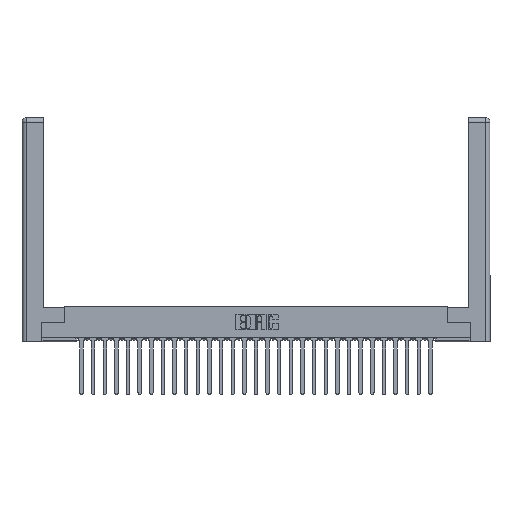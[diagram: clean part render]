
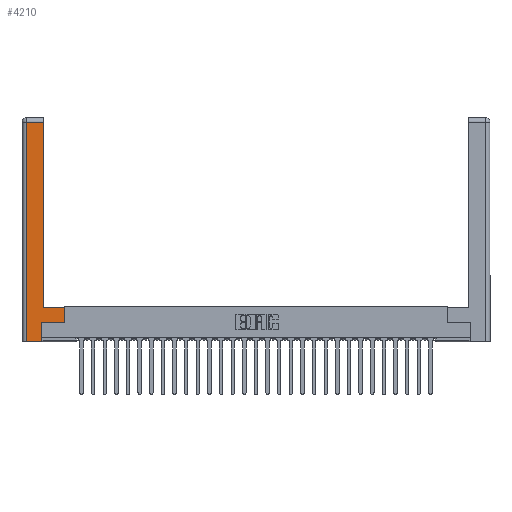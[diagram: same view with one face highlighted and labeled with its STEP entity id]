
A CAD part, top view. The second image highlights one B-rep face of the part: STEP entity #4210.
In plain terms, the highlighted planar face has unit normal (0, 0, 1).
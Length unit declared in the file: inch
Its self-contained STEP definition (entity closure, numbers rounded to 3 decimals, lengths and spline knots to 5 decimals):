
#70 = CARTESIAN_POINT ( 'NONE',  ( 0.265, 0.245, 0. ) ) ;
#2026 = VERTEX_POINT ( 'NONE', #13066 ) ;
#2147 = LINE ( 'NONE', #11250, #27259 ) ;
#2596 = DIRECTION ( 'NONE',  ( -1., 0., 0. ) ) ;
#3195 = ORIENTED_EDGE ( 'NONE', *, *, #26082, .T. ) ;
#3991 = EDGE_CURVE ( 'NONE', #13642, #24415, #12221, .T. ) ;
#4210 = ADVANCED_FACE ( 'NONE', ( #15897 ), #30263, .F. ) ;
#4246 = VECTOR ( 'NONE', #17911, 39.37008 ) ;
#5346 = VECTOR ( 'NONE', #6968, 39.37008 ) ;
#6277 = VERTEX_POINT ( 'NONE', #70 ) ;
#6968 = DIRECTION ( 'NONE',  ( 0., 1., 0. ) ) ;
#7198 = DIRECTION ( 'NONE',  ( 1., 0., 0. ) ) ;
#8032 = EDGE_CURVE ( 'NONE', #24415, #6277, #14075, .T. ) ;
#8377 = VERTEX_POINT ( 'NONE', #27374 ) ;
#8757 = LINE ( 'NONE', #20381, #4246 ) ;
#9289 = CARTESIAN_POINT ( 'NONE',  ( 0.265, 0., 0. ) ) ;
#9421 = VECTOR ( 'NONE', #11457, 39.37008 ) ;
#10796 = ORIENTED_EDGE ( 'NONE', *, *, #13931, .T. ) ;
#11250 = CARTESIAN_POINT ( 'NONE',  ( 0.0615, 0., 0. ) ) ;
#11457 = DIRECTION ( 'NONE',  ( 0., 1., 0. ) ) ;
#12221 = LINE ( 'NONE', #9289, #17261 ) ;
#12653 = VERTEX_POINT ( 'NONE', #21847 ) ;
#12697 = CARTESIAN_POINT ( 'NONE',  ( 0.295, 3., 0. ) ) ;
#12807 = AXIS2_PLACEMENT_3D ( 'NONE', #29969, #27659, #16195 ) ;
#13066 = CARTESIAN_POINT ( 'NONE',  ( 0.295, 2.94, 0. ) ) ;
#13238 = CARTESIAN_POINT ( 'NONE',  ( 0.565, 0.245, 0. ) ) ;
#13642 = VERTEX_POINT ( 'NONE', #19598 ) ;
#13931 = EDGE_CURVE ( 'NONE', #6277, #22882, #23302, .T. ) ;
#14075 = LINE ( 'NONE', #28162, #5346 ) ;
#14352 = VECTOR ( 'NONE', #21273, 39.37008 ) ;
#15060 = EDGE_CURVE ( 'NONE', #12653, #30357, #8757, .T. ) ;
#15392 = ORIENTED_EDGE ( 'NONE', *, *, #19309, .T. ) ;
#15897 = FACE_OUTER_BOUND ( 'NONE', #22704, .T. ) ;
#16195 = DIRECTION ( 'NONE',  ( -1., 0., 0. ) ) ;
#17261 = VECTOR ( 'NONE', #21227, 39.37008 ) ;
#17666 = LINE ( 'NONE', #12697, #14352 ) ;
#17911 = DIRECTION ( 'NONE',  ( -1., 0., 0. ) ) ;
#18518 = ORIENTED_EDGE ( 'NONE', *, *, #15060, .T. ) ;
#18718 = ORIENTED_EDGE ( 'NONE', *, *, #21838, .T. ) ;
#18902 = LINE ( 'NONE', #23404, #9421 ) ;
#19309 = EDGE_CURVE ( 'NONE', #2026, #8377, #23787, .T. ) ;
#19598 = CARTESIAN_POINT ( 'NONE',  ( 0.0615, 0., 0. ) ) ;
#20381 = CARTESIAN_POINT ( 'NONE',  ( 0.295, 0.45, 0. ) ) ;
#20467 = CARTESIAN_POINT ( 'NONE',  ( 0.265, 0., 0. ) ) ;
#21227 = DIRECTION ( 'NONE',  ( 1., 0., 0. ) ) ;
#21273 = DIRECTION ( 'NONE',  ( 0., 1., 0. ) ) ;
#21838 = EDGE_CURVE ( 'NONE', #30357, #2026, #17666, .T. ) ;
#21847 = CARTESIAN_POINT ( 'NONE',  ( 0.565, 0.45, 0. ) ) ;
#22194 = CARTESIAN_POINT ( 'NONE',  ( 0.0615, 2.94, 0. ) ) ;
#22704 = EDGE_LOOP ( 'NONE', ( #18718, #15392, #29010, #28416, #23493, #10796, #3195, #18518 ) ) ;
#22882 = VERTEX_POINT ( 'NONE', #13238 ) ;
#23302 = LINE ( 'NONE', #28527, #24413 ) ;
#23404 = CARTESIAN_POINT ( 'NONE',  ( 0.565, 0.45, 0. ) ) ;
#23493 = ORIENTED_EDGE ( 'NONE', *, *, #8032, .T. ) ;
#23787 = LINE ( 'NONE', #22194, #25599 ) ;
#24406 = CARTESIAN_POINT ( 'NONE',  ( 0.295, 0.45, 0. ) ) ;
#24413 = VECTOR ( 'NONE', #7198, 39.37008 ) ;
#24415 = VERTEX_POINT ( 'NONE', #20467 ) ;
#25358 = DIRECTION ( 'NONE',  ( 0., -1., 0. ) ) ;
#25599 = VECTOR ( 'NONE', #2596, 39.37008 ) ;
#26082 = EDGE_CURVE ( 'NONE', #22882, #12653, #18902, .T. ) ;
#27259 = VECTOR ( 'NONE', #25358, 39.37008 ) ;
#27374 = CARTESIAN_POINT ( 'NONE',  ( 0.0615, 2.94, 0. ) ) ;
#27659 = DIRECTION ( 'NONE',  ( 0., 0., -1. ) ) ;
#28162 = CARTESIAN_POINT ( 'NONE',  ( 0.265, 0.245, 0. ) ) ;
#28305 = EDGE_CURVE ( 'NONE', #8377, #13642, #2147, .T. ) ;
#28416 = ORIENTED_EDGE ( 'NONE', *, *, #3991, .T. ) ;
#28527 = CARTESIAN_POINT ( 'NONE',  ( 0.565, 0.245, 0. ) ) ;
#29010 = ORIENTED_EDGE ( 'NONE', *, *, #28305, .T. ) ;
#29969 = CARTESIAN_POINT ( 'NONE',  ( 0., 0., 0. ) ) ;
#30263 = PLANE ( 'NONE',  #12807 ) ;
#30357 = VERTEX_POINT ( 'NONE', #24406 ) ;
